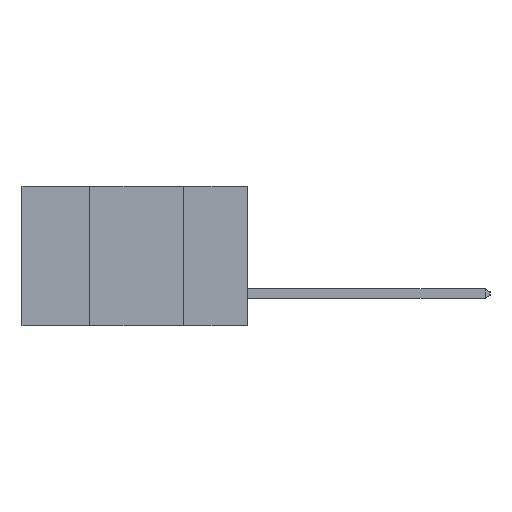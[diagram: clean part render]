
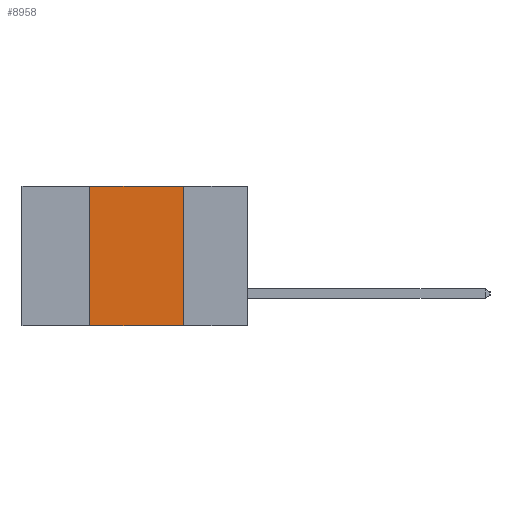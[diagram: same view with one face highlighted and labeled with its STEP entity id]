
A CAD part, left-side view. The second image highlights one B-rep face of the part: STEP entity #8958.
In plain terms, the highlighted planar face has unit normal (-1, 0, 0).
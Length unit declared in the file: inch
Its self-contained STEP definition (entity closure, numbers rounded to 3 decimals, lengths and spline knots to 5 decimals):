
#2362 = DIRECTION ( 'NONE',  ( 0., 0., -1. ) ) ;
#4048 = CARTESIAN_POINT ( 'NONE',  ( 0., 0.17, -0.37 ) ) ;
#4104 = AXIS2_PLACEMENT_3D ( 'NONE', #7345, #17406, #2362 ) ;
#4312 = CARTESIAN_POINT ( 'NONE',  ( 0., 0.42, -0.37 ) ) ;
#4644 = EDGE_CURVE ( 'NONE', #25491, #20402, #25035, .T. ) ;
#5297 = DIRECTION ( 'NONE',  ( 0., 0., 1. ) ) ;
#5687 = VECTOR ( 'NONE', #18279, 39.37008 ) ;
#5734 = DIRECTION ( 'NONE',  ( 0., -1., 0. ) ) ;
#5781 = CARTESIAN_POINT ( 'NONE',  ( 0., 0.42, 0. ) ) ;
#6168 = CARTESIAN_POINT ( 'NONE',  ( 0., 0.42, 0. ) ) ;
#7345 = CARTESIAN_POINT ( 'NONE',  ( 0., 0.6, 0. ) ) ;
#8958 = ADVANCED_FACE ( 'NONE', ( #27854 ), #14940, .F. ) ;
#10710 = EDGE_LOOP ( 'NONE', ( #12390, #27034, #31712, #11740 ) ) ;
#11229 = VECTOR ( 'NONE', #5297, 39.37008 ) ;
#11472 = DIRECTION ( 'NONE',  ( 0., 0., -1. ) ) ;
#11740 = ORIENTED_EDGE ( 'NONE', *, *, #26842, .T. ) ;
#12390 = ORIENTED_EDGE ( 'NONE', *, *, #13607, .F. ) ;
#12903 = CARTESIAN_POINT ( 'NONE',  ( 0., 0.17, 0. ) ) ;
#13607 = EDGE_CURVE ( 'NONE', #15297, #26096, #15802, .T. ) ;
#13988 = CARTESIAN_POINT ( 'NONE',  ( 0., 0.17, 0. ) ) ;
#14068 = EDGE_CURVE ( 'NONE', #20402, #15297, #25452, .T. ) ;
#14149 = VECTOR ( 'NONE', #5734, 39.37008 ) ;
#14940 = PLANE ( 'NONE',  #4104 ) ;
#14943 = LINE ( 'NONE', #15773, #14149 ) ;
#15297 = VERTEX_POINT ( 'NONE', #12903 ) ;
#15773 = CARTESIAN_POINT ( 'NONE',  ( 0., 0.6, -0.37 ) ) ;
#15798 = CARTESIAN_POINT ( 'NONE',  ( 0., 0.6, 0. ) ) ;
#15802 = LINE ( 'NONE', #13988, #21487 ) ;
#17406 = DIRECTION ( 'NONE',  ( 1., 0., 0. ) ) ;
#18279 = DIRECTION ( 'NONE',  ( 0., -1., 0. ) ) ;
#20402 = VERTEX_POINT ( 'NONE', #6168 ) ;
#21487 = VECTOR ( 'NONE', #11472, 39.37008 ) ;
#25035 = LINE ( 'NONE', #5781, #11229 ) ;
#25452 = LINE ( 'NONE', #15798, #5687 ) ;
#25491 = VERTEX_POINT ( 'NONE', #4312 ) ;
#26096 = VERTEX_POINT ( 'NONE', #4048 ) ;
#26842 = EDGE_CURVE ( 'NONE', #25491, #26096, #14943, .T. ) ;
#27034 = ORIENTED_EDGE ( 'NONE', *, *, #14068, .F. ) ;
#27854 = FACE_OUTER_BOUND ( 'NONE', #10710, .T. ) ;
#31712 = ORIENTED_EDGE ( 'NONE', *, *, #4644, .F. ) ;
